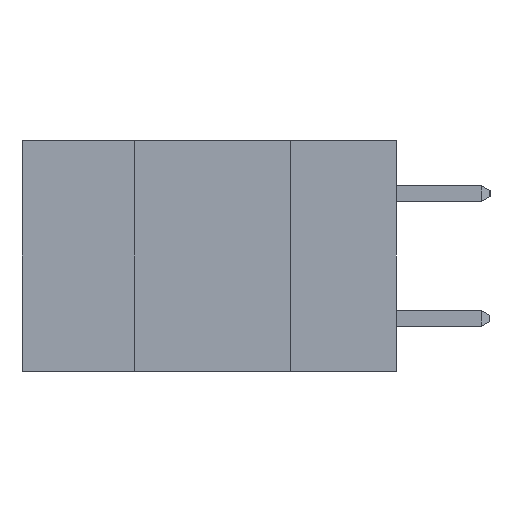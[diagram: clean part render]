
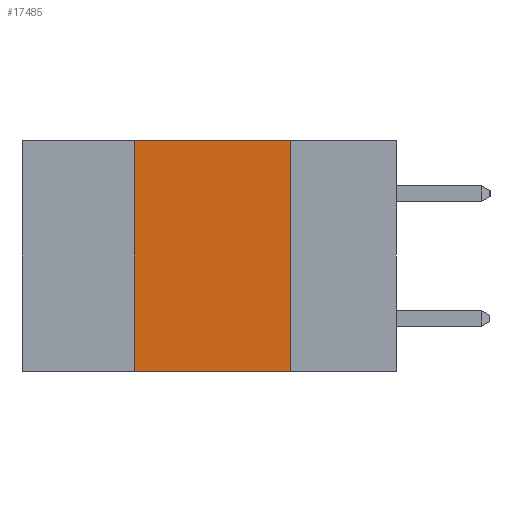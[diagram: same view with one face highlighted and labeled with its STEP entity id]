
A CAD part, left-side view. The second image highlights one B-rep face of the part: STEP entity #17485.
In plain terms, the highlighted planar face has unit normal (-1, 0, 0).
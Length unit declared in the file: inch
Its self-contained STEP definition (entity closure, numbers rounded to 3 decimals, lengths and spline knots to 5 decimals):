
#312 = LINE ( 'NONE', #2120, #18150 ) ;
#506 = ORIENTED_EDGE ( 'NONE', *, *, #11475, .T. ) ;
#877 = DIRECTION ( 'NONE',  ( 0., 0., -1. ) ) ;
#1912 = CARTESIAN_POINT ( 'NONE',  ( 0., 0.42, -0.37 ) ) ;
#2120 = CARTESIAN_POINT ( 'NONE',  ( 0., 0.42, -0.37 ) ) ;
#2171 = PLANE ( 'NONE',  #10506 ) ;
#2183 = LINE ( 'NONE', #7212, #18009 ) ;
#6240 = ORIENTED_EDGE ( 'NONE', *, *, #7520, .F. ) ;
#6901 = DIRECTION ( 'NONE',  ( 0., 0., -1. ) ) ;
#7212 = CARTESIAN_POINT ( 'NONE',  ( 0., 0.17, -0.37 ) ) ;
#7520 = EDGE_CURVE ( 'NONE', #9559, #15325, #2183, .T. ) ;
#7676 = CARTESIAN_POINT ( 'NONE',  ( 0., 0.17, -0.37 ) ) ;
#9559 = VERTEX_POINT ( 'NONE', #18331 ) ;
#10163 = DIRECTION ( 'NONE',  ( 0., 0., 1. ) ) ;
#10494 = ORIENTED_EDGE ( 'NONE', *, *, #20625, .F. ) ;
#10506 = AXIS2_PLACEMENT_3D ( 'NONE', #13529, #16772, #6901 ) ;
#10965 = EDGE_LOOP ( 'NONE', ( #6240, #10494, #13856, #506 ) ) ;
#11418 = VECTOR ( 'NONE', #12733, 39.37008 ) ;
#11475 = EDGE_CURVE ( 'NONE', #20379, #15325, #17687, .T. ) ;
#12733 = DIRECTION ( 'NONE',  ( 0., -1., 0. ) ) ;
#13424 = FACE_OUTER_BOUND ( 'NONE', #10965, .T. ) ;
#13529 = CARTESIAN_POINT ( 'NONE',  ( 0., 0.6, 0. ) ) ;
#13856 = ORIENTED_EDGE ( 'NONE', *, *, #20470, .F. ) ;
#14003 = DIRECTION ( 'NONE',  ( 0., -1., 0. ) ) ;
#14109 = CARTESIAN_POINT ( 'NONE',  ( 0., 0.6, 0. ) ) ;
#15325 = VERTEX_POINT ( 'NONE', #7676 ) ;
#16087 = CARTESIAN_POINT ( 'NONE',  ( 0., 0.6, -0.37 ) ) ;
#16772 = DIRECTION ( 'NONE',  ( 1., 0., 0. ) ) ;
#17451 = VECTOR ( 'NONE', #14003, 39.37008 ) ;
#17485 = ADVANCED_FACE ( 'NONE', ( #13424 ), #2171, .F. ) ;
#17687 = LINE ( 'NONE', #16087, #11418 ) ;
#18009 = VECTOR ( 'NONE', #877, 39.37008 ) ;
#18150 = VECTOR ( 'NONE', #10163, 39.37008 ) ;
#18331 = CARTESIAN_POINT ( 'NONE',  ( 0., 0.17, 0. ) ) ;
#18527 = CARTESIAN_POINT ( 'NONE',  ( 0., 0.42, 0. ) ) ;
#18936 = LINE ( 'NONE', #14109, #17451 ) ;
#20379 = VERTEX_POINT ( 'NONE', #1912 ) ;
#20470 = EDGE_CURVE ( 'NONE', #20379, #20498, #312, .T. ) ;
#20498 = VERTEX_POINT ( 'NONE', #18527 ) ;
#20625 = EDGE_CURVE ( 'NONE', #20498, #9559, #18936, .T. ) ;
